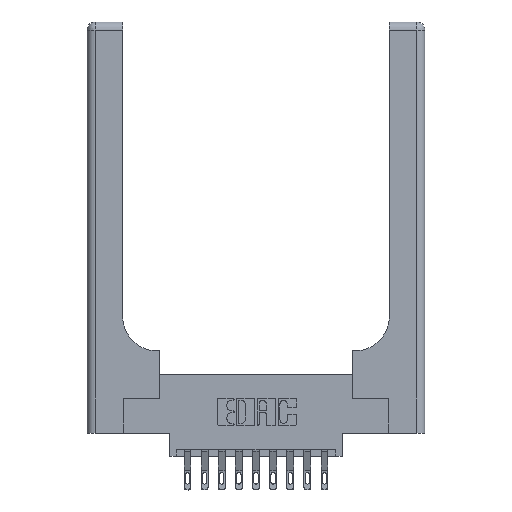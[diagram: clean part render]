
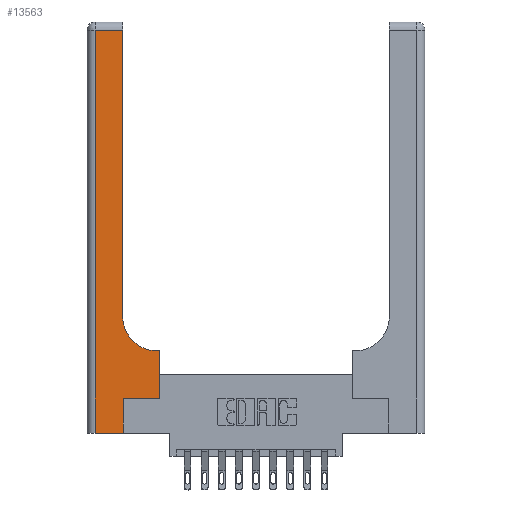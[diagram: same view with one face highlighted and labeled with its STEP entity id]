
A CAD part, top view. The second image highlights one B-rep face of the part: STEP entity #13563.
In plain terms, the highlighted planar face has unit normal (0, 0, 1).
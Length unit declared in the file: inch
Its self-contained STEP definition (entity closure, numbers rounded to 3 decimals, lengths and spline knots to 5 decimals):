
#310 = CARTESIAN_POINT ( 'NONE',  ( 0.06, 3., 0.37 ) ) ;
#427 = VECTOR ( 'NONE', #3234, 39.37008 ) ;
#447 = ORIENTED_EDGE ( 'NONE', *, *, #11553, .T. ) ;
#538 = CARTESIAN_POINT ( 'NONE',  ( 0.265, 0.25, 0.37 ) ) ;
#741 = DIRECTION ( 'NONE',  ( 0., 1., 0. ) ) ;
#1283 = VECTOR ( 'NONE', #7760, 39.37008 ) ;
#1411 = CARTESIAN_POINT ( 'NONE',  ( 0.51, 0.85, 0.37 ) ) ;
#1600 = ORIENTED_EDGE ( 'NONE', *, *, #4751, .T. ) ;
#1614 = CIRCLE ( 'NONE', #1968, 0.25 ) ;
#1942 = CARTESIAN_POINT ( 'NONE',  ( 0.06, 2.94, 0.37 ) ) ;
#1968 = AXIS2_PLACEMENT_3D ( 'NONE', #1411, #10062, #2663 ) ;
#2455 = CARTESIAN_POINT ( 'NONE',  ( 0.51, 0.6, 0.37 ) ) ;
#2467 = VECTOR ( 'NONE', #741, 39.37008 ) ;
#2663 = DIRECTION ( 'NONE',  ( 1., 0., 0. ) ) ;
#2775 = VERTEX_POINT ( 'NONE', #14799 ) ;
#2832 = PLANE ( 'NONE',  #3627 ) ;
#3234 = DIRECTION ( 'NONE',  ( 1., 0., 0. ) ) ;
#3331 = CARTESIAN_POINT ( 'NONE',  ( 0.265, 0., 0.37 ) ) ;
#3440 = EDGE_CURVE ( 'NONE', #6371, #4184, #12516, .T. ) ;
#3627 = AXIS2_PLACEMENT_3D ( 'NONE', #4020, #12673, #5322 ) ;
#3696 = VERTEX_POINT ( 'NONE', #3331 ) ;
#3719 = ORIENTED_EDGE ( 'NONE', *, *, #3440, .T. ) ;
#3869 = DIRECTION ( 'NONE',  ( 1., 0., 0. ) ) ;
#3907 = LINE ( 'NONE', #5084, #7608 ) ;
#3970 = VERTEX_POINT ( 'NONE', #8764 ) ;
#4020 = CARTESIAN_POINT ( 'NONE',  ( 0., 3., 0.37 ) ) ;
#4051 = VERTEX_POINT ( 'NONE', #4174 ) ;
#4139 = VERTEX_POINT ( 'NONE', #538 ) ;
#4174 = CARTESIAN_POINT ( 'NONE',  ( 0.26, 0.85, 0.37 ) ) ;
#4184 = VERTEX_POINT ( 'NONE', #1942 ) ;
#4423 = CARTESIAN_POINT ( 'NONE',  ( 0.26, 3., 0.37 ) ) ;
#4751 = EDGE_CURVE ( 'NONE', #4184, #3970, #14385, .T. ) ;
#5084 = CARTESIAN_POINT ( 'NONE',  ( 0.528, 0.25, 0.37 ) ) ;
#5322 = DIRECTION ( 'NONE',  ( -1., 0., 0. ) ) ;
#6371 = VERTEX_POINT ( 'NONE', #13201 ) ;
#6379 = EDGE_CURVE ( 'NONE', #9208, #7520, #8393, .T. ) ;
#6410 = LINE ( 'NONE', #10024, #15819 ) ;
#6540 = LINE ( 'NONE', #10339, #13035 ) ;
#6648 = EDGE_CURVE ( 'NONE', #7520, #4051, #1614, .T. ) ;
#6816 = EDGE_LOOP ( 'NONE', ( #7605, #3719, #1600, #15469, #447, #9572, #7086, #11488, #15141 ) ) ;
#7086 = ORIENTED_EDGE ( 'NONE', *, *, #15253, .T. ) ;
#7190 = CARTESIAN_POINT ( 'NONE',  ( 0.528, 0.6, 0.37 ) ) ;
#7520 = VERTEX_POINT ( 'NONE', #2455 ) ;
#7605 = ORIENTED_EDGE ( 'NONE', *, *, #11155, .T. ) ;
#7608 = VECTOR ( 'NONE', #9840, 39.37008 ) ;
#7760 = DIRECTION ( 'NONE',  ( 0., -1., 0. ) ) ;
#7845 = DIRECTION ( 'NONE',  ( -1., 0., 0. ) ) ;
#8268 = LINE ( 'NONE', #4423, #2467 ) ;
#8393 = LINE ( 'NONE', #14446, #11276 ) ;
#8764 = CARTESIAN_POINT ( 'NONE',  ( 0.06, 0., 0.37 ) ) ;
#9208 = VERTEX_POINT ( 'NONE', #7190 ) ;
#9350 = FACE_OUTER_BOUND ( 'NONE', #6816, .T. ) ;
#9387 = EDGE_CURVE ( 'NONE', #3970, #3696, #6410, .T. ) ;
#9572 = ORIENTED_EDGE ( 'NONE', *, *, #14243, .T. ) ;
#9840 = DIRECTION ( 'NONE',  ( 0., 1., 0. ) ) ;
#10024 = CARTESIAN_POINT ( 'NONE',  ( 0., 0., 0.37 ) ) ;
#10062 = DIRECTION ( 'NONE',  ( 0., 0., -1. ) ) ;
#10244 = CARTESIAN_POINT ( 'NONE',  ( 0., 2.94, 0.37 ) ) ;
#10339 = CARTESIAN_POINT ( 'NONE',  ( 0.265, 0., 0.37 ) ) ;
#11155 = EDGE_CURVE ( 'NONE', #4051, #6371, #8268, .T. ) ;
#11276 = VECTOR ( 'NONE', #15691, 39.37008 ) ;
#11488 = ORIENTED_EDGE ( 'NONE', *, *, #6379, .T. ) ;
#11553 = EDGE_CURVE ( 'NONE', #3696, #4139, #6540, .T. ) ;
#11571 = DIRECTION ( 'NONE',  ( 0., 1., 0. ) ) ;
#12516 = LINE ( 'NONE', #10244, #15007 ) ;
#12673 = DIRECTION ( 'NONE',  ( 0., 0., -1. ) ) ;
#13035 = VECTOR ( 'NONE', #11571, 39.37008 ) ;
#13201 = CARTESIAN_POINT ( 'NONE',  ( 0.26, 2.94, 0.37 ) ) ;
#13563 = ADVANCED_FACE ( 'NONE', ( #9350 ), #2832, .F. ) ;
#13923 = LINE ( 'NONE', #15492, #427 ) ;
#14243 = EDGE_CURVE ( 'NONE', #4139, #2775, #13923, .T. ) ;
#14385 = LINE ( 'NONE', #310, #1283 ) ;
#14446 = CARTESIAN_POINT ( 'NONE',  ( 0.26, 0.6, 0.37 ) ) ;
#14799 = CARTESIAN_POINT ( 'NONE',  ( 0.528, 0.25, 0.37 ) ) ;
#15007 = VECTOR ( 'NONE', #7845, 39.37008 ) ;
#15141 = ORIENTED_EDGE ( 'NONE', *, *, #6648, .T. ) ;
#15253 = EDGE_CURVE ( 'NONE', #2775, #9208, #3907, .T. ) ;
#15469 = ORIENTED_EDGE ( 'NONE', *, *, #9387, .T. ) ;
#15492 = CARTESIAN_POINT ( 'NONE',  ( 0.265, 0.25, 0.37 ) ) ;
#15691 = DIRECTION ( 'NONE',  ( -1., 0., 0. ) ) ;
#15819 = VECTOR ( 'NONE', #3869, 39.37008 ) ;
